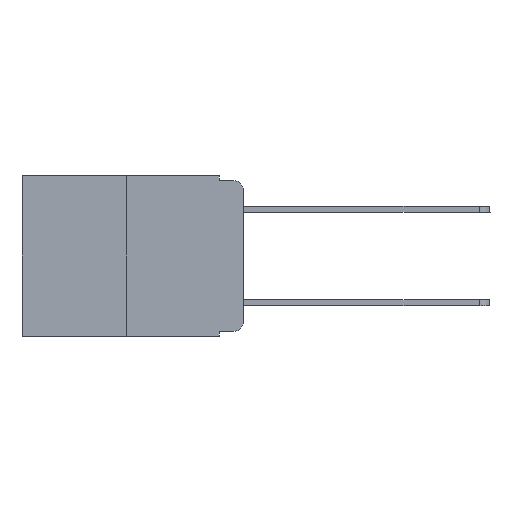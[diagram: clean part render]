
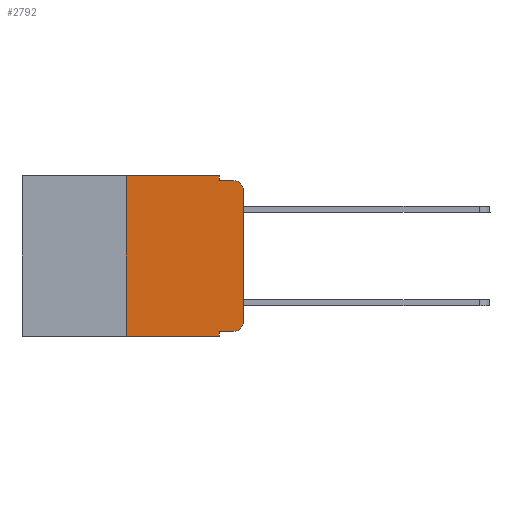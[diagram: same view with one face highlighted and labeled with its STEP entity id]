
A CAD part, left-side view. The second image highlights one B-rep face of the part: STEP entity #2792.
In plain terms, the highlighted planar face has unit normal (-1, 0, 0).
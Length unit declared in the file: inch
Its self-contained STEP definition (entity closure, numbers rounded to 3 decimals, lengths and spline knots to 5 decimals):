
#7 = VECTOR ( 'NONE', #1954, 39.37008 ) ;
#12 = VECTOR ( 'NONE', #13386, 39.37008 ) ;
#71 = ORIENTED_EDGE ( 'NONE', *, *, #6928, .F. ) ;
#293 = VERTEX_POINT ( 'NONE', #5989 ) ;
#711 = DIRECTION ( 'NONE',  ( 0., 0., 1. ) ) ;
#813 = CARTESIAN_POINT ( 'NONE',  ( 0., 0.051, 0. ) ) ;
#874 = EDGE_CURVE ( 'NONE', #11899, #6849, #1412, .T. ) ;
#917 = CIRCLE ( 'NONE', #5207, 0.02 ) ;
#1204 = CARTESIAN_POINT ( 'NONE',  ( 0., 0.051, -0.333 ) ) ;
#1412 = CIRCLE ( 'NONE', #6180, 0.02 ) ;
#1941 = DIRECTION ( 'NONE',  ( 0., 0., -1. ) ) ;
#1954 = DIRECTION ( 'NONE',  ( 0., -1., 0. ) ) ;
#2135 = CARTESIAN_POINT ( 'NONE',  ( 0., 0.02, -0.313 ) ) ;
#2762 = DIRECTION ( 'NONE',  ( 0., 0., -1. ) ) ;
#2792 = ADVANCED_FACE ( 'NONE', ( #6875 ), #10932, .F. ) ;
#2817 = ORIENTED_EDGE ( 'NONE', *, *, #5585, .F. ) ;
#2831 = ORIENTED_EDGE ( 'NONE', *, *, #9142, .F. ) ;
#2899 = EDGE_CURVE ( 'NONE', #8482, #3905, #12608, .T. ) ;
#3009 = CARTESIAN_POINT ( 'NONE',  ( 0., 0.02, -0.03 ) ) ;
#3019 = LINE ( 'NONE', #11675, #7 ) ;
#3241 = EDGE_CURVE ( 'NONE', #6322, #293, #917, .T. ) ;
#3379 = DIRECTION ( 'NONE',  ( 0., 0., 1. ) ) ;
#3905 = VERTEX_POINT ( 'NONE', #10650 ) ;
#4049 = ORIENTED_EDGE ( 'NONE', *, *, #4839, .T. ) ;
#4167 = LINE ( 'NONE', #8510, #7940 ) ;
#4457 = VERTEX_POINT ( 'NONE', #10102 ) ;
#4525 = EDGE_CURVE ( 'NONE', #6282, #11899, #4637, .T. ) ;
#4637 = LINE ( 'NONE', #1204, #12 ) ;
#4728 = VECTOR ( 'NONE', #3379, 39.37008 ) ;
#4839 = EDGE_CURVE ( 'NONE', #6849, #6322, #13029, .T. ) ;
#4892 = VERTEX_POINT ( 'NONE', #5577 ) ;
#4903 = CARTESIAN_POINT ( 'NONE',  ( 0., 0.473, 0. ) ) ;
#4938 = LINE ( 'NONE', #13614, #12389 ) ;
#5158 = VECTOR ( 'NONE', #5995, 39.37008 ) ;
#5207 = AXIS2_PLACEMENT_3D ( 'NONE', #3009, #9045, #1941 ) ;
#5214 = EDGE_CURVE ( 'NONE', #6282, #7591, #7276, .T. ) ;
#5577 = CARTESIAN_POINT ( 'NONE',  ( 0., 0.25, -0.343 ) ) ;
#5585 = EDGE_CURVE ( 'NONE', #3905, #293, #4167, .T. ) ;
#5989 = CARTESIAN_POINT ( 'NONE',  ( 0., 0.02, -0.01 ) ) ;
#5995 = DIRECTION ( 'NONE',  ( 0., -1., 0. ) ) ;
#6180 = AXIS2_PLACEMENT_3D ( 'NONE', #2135, #13841, #6408 ) ;
#6282 = VERTEX_POINT ( 'NONE', #11082 ) ;
#6322 = VERTEX_POINT ( 'NONE', #7893 ) ;
#6408 = DIRECTION ( 'NONE',  ( 0., 0., -1. ) ) ;
#6849 = VERTEX_POINT ( 'NONE', #8284 ) ;
#6875 = FACE_OUTER_BOUND ( 'NONE', #13236, .T. ) ;
#6928 = EDGE_CURVE ( 'NONE', #4892, #4457, #4938, .T. ) ;
#7156 = ORIENTED_EDGE ( 'NONE', *, *, #4525, .T. ) ;
#7239 = VECTOR ( 'NONE', #2762, 39.37008 ) ;
#7276 = LINE ( 'NONE', #813, #9519 ) ;
#7591 = VERTEX_POINT ( 'NONE', #8890 ) ;
#7620 = ORIENTED_EDGE ( 'NONE', *, *, #5214, .F. ) ;
#7750 = CARTESIAN_POINT ( 'NONE',  ( 0., 0.02, -0.333 ) ) ;
#7832 = ORIENTED_EDGE ( 'NONE', *, *, #3241, .T. ) ;
#7893 = CARTESIAN_POINT ( 'NONE',  ( 0., 0., -0.03 ) ) ;
#7940 = VECTOR ( 'NONE', #12834, 39.37008 ) ;
#7941 = DIRECTION ( 'NONE',  ( 0., 0., -1. ) ) ;
#8043 = ORIENTED_EDGE ( 'NONE', *, *, #10598, .T. ) ;
#8229 = CARTESIAN_POINT ( 'NONE',  ( 0., 0.051, 0. ) ) ;
#8284 = CARTESIAN_POINT ( 'NONE',  ( 0., 0., -0.313 ) ) ;
#8482 = VERTEX_POINT ( 'NONE', #8860 ) ;
#8510 = CARTESIAN_POINT ( 'NONE',  ( 0., 0.051, -0.01 ) ) ;
#8654 = ORIENTED_EDGE ( 'NONE', *, *, #874, .T. ) ;
#8860 = CARTESIAN_POINT ( 'NONE',  ( 0., 0.051, 0. ) ) ;
#8890 = CARTESIAN_POINT ( 'NONE',  ( 0., 0.051, -0.343 ) ) ;
#9045 = DIRECTION ( 'NONE',  ( -1., 0., 0. ) ) ;
#9066 = DIRECTION ( 'NONE',  ( 0., 0., -1. ) ) ;
#9142 = EDGE_CURVE ( 'NONE', #4457, #8482, #12431, .T. ) ;
#9519 = VECTOR ( 'NONE', #9066, 39.37008 ) ;
#9833 = CARTESIAN_POINT ( 'NONE',  ( 0., 0., 0. ) ) ;
#10102 = CARTESIAN_POINT ( 'NONE',  ( 0., 0.25, 0. ) ) ;
#10598 = EDGE_CURVE ( 'NONE', #4892, #7591, #3019, .T. ) ;
#10650 = CARTESIAN_POINT ( 'NONE',  ( 0., 0.051, -0.01 ) ) ;
#10825 = ORIENTED_EDGE ( 'NONE', *, *, #2899, .F. ) ;
#10932 = PLANE ( 'NONE',  #12916 ) ;
#11082 = CARTESIAN_POINT ( 'NONE',  ( 0., 0.051, -0.333 ) ) ;
#11675 = CARTESIAN_POINT ( 'NONE',  ( 0., 0.473, -0.343 ) ) ;
#11899 = VERTEX_POINT ( 'NONE', #7750 ) ;
#12120 = DIRECTION ( 'NONE',  ( 1., 0., 0. ) ) ;
#12389 = VECTOR ( 'NONE', #711, 39.37008 ) ;
#12431 = LINE ( 'NONE', #4903, #5158 ) ;
#12608 = LINE ( 'NONE', #8229, #7239 ) ;
#12834 = DIRECTION ( 'NONE',  ( 0., -1., 0. ) ) ;
#12916 = AXIS2_PLACEMENT_3D ( 'NONE', #13128, #12120, #7941 ) ;
#13029 = LINE ( 'NONE', #9833, #4728 ) ;
#13128 = CARTESIAN_POINT ( 'NONE',  ( 0., 0.473, 0. ) ) ;
#13236 = EDGE_LOOP ( 'NONE', ( #4049, #7832, #2817, #10825, #2831, #71, #8043, #7620, #7156, #8654 ) ) ;
#13386 = DIRECTION ( 'NONE',  ( 0., -1., 0. ) ) ;
#13614 = CARTESIAN_POINT ( 'NONE',  ( 0., 0.25, 0. ) ) ;
#13841 = DIRECTION ( 'NONE',  ( -1., 0., 0. ) ) ;
